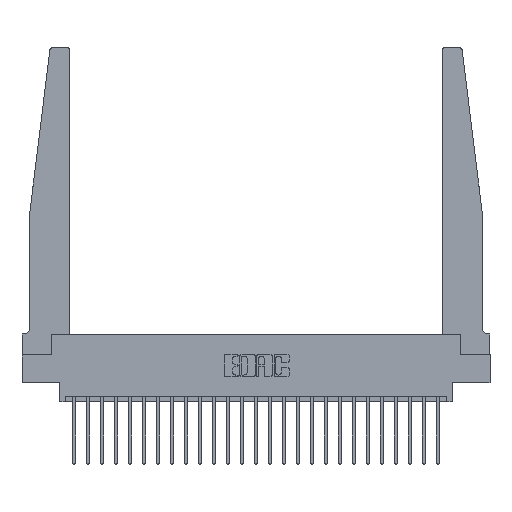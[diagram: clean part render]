
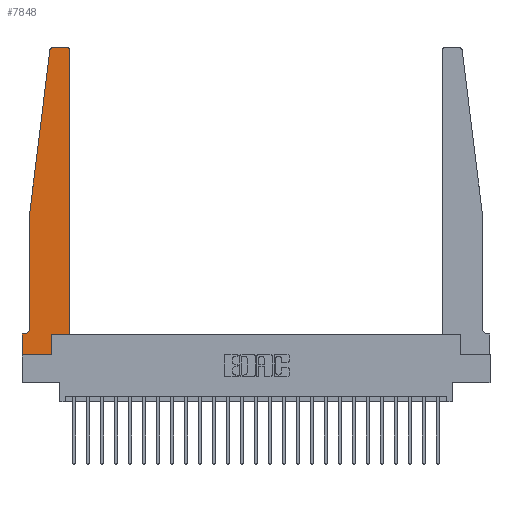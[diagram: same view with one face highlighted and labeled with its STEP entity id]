
A CAD part, top view. The second image highlights one B-rep face of the part: STEP entity #7848.
In plain terms, the highlighted planar face has unit normal (0, 0, 1).
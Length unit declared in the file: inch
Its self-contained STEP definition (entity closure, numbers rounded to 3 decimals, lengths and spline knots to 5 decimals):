
#26 = DIRECTION ( 'NONE',  ( -1., 0., 0. ) ) ;
#931 = LINE ( 'NONE', #16003, #6607 ) ;
#1035 = CARTESIAN_POINT ( 'NONE',  ( 0.065, 1.25, 0.37 ) ) ;
#1192 = VERTEX_POINT ( 'NONE', #6724 ) ;
#1644 = VERTEX_POINT ( 'NONE', #19630 ) ;
#2018 = AXIS2_PLACEMENT_3D ( 'NONE', #3687, #19014, #7598 ) ;
#2164 = CARTESIAN_POINT ( 'NONE',  ( 0.065, 0.1875, 0.37 ) ) ;
#2196 = CARTESIAN_POINT ( 'NONE',  ( 0., 0.1875, 0.37 ) ) ;
#2703 = CARTESIAN_POINT ( 'NONE',  ( 0.2605, 0.18, 0.37 ) ) ;
#3078 = VECTOR ( 'NONE', #17580, 39.37008 ) ;
#3254 = DIRECTION ( 'NONE',  ( 1., 0., 0. ) ) ;
#3283 = LINE ( 'NONE', #2164, #17925 ) ;
#3306 = CARTESIAN_POINT ( 'NONE',  ( 0.27653, 2.72, 0.37 ) ) ;
#3687 = CARTESIAN_POINT ( 'NONE',  ( 0., 0.1875, 0.37 ) ) ;
#3842 = VECTOR ( 'NONE', #23793, 39.37008 ) ;
#3896 = VERTEX_POINT ( 'NONE', #21980 ) ;
#3929 = VECTOR ( 'NONE', #10634, 39.37008 ) ;
#4028 = VERTEX_POINT ( 'NONE', #14715 ) ;
#4054 = DIRECTION ( 'NONE',  ( 0., 0., 1. ) ) ;
#4453 = ORIENTED_EDGE ( 'NONE', *, *, #22277, .T. ) ;
#4583 = CIRCLE ( 'NONE', #8729, 0.05 ) ;
#4619 = EDGE_CURVE ( 'NONE', #16346, #22479, #21189, .T. ) ;
#4813 = VERTEX_POINT ( 'NONE', #20876 ) ;
#4821 = LINE ( 'NONE', #10962, #23227 ) ;
#4935 = CIRCLE ( 'NONE', #9643, 0.03 ) ;
#4968 = CIRCLE ( 'NONE', #6593, 0.03 ) ;
#5007 = VERTEX_POINT ( 'NONE', #8241 ) ;
#5050 = ORIENTED_EDGE ( 'NONE', *, *, #11134, .T. ) ;
#5052 = ORIENTED_EDGE ( 'NONE', *, *, #17417, .T. ) ;
#5088 = CARTESIAN_POINT ( 'NONE',  ( 0.425, 2.72, 0.37 ) ) ;
#5091 = EDGE_CURVE ( 'NONE', #22479, #13939, #931, .T. ) ;
#5223 = DIRECTION ( 'NONE',  ( 1., 0., 0. ) ) ;
#5710 = CARTESIAN_POINT ( 'NONE',  ( 0.425, 0.18, 0.37 ) ) ;
#5969 = ORIENTED_EDGE ( 'NONE', *, *, #22006, .T. ) ;
#6244 = ORIENTED_EDGE ( 'NONE', *, *, #21974, .T. ) ;
#6593 = AXIS2_PLACEMENT_3D ( 'NONE', #3306, #16664, #5223 ) ;
#6607 = VECTOR ( 'NONE', #17930, 39.37008 ) ;
#6724 = CARTESIAN_POINT ( 'NONE',  ( 0.24675, 2.72367, 0.37 ) ) ;
#6766 = CARTESIAN_POINT ( 'NONE',  ( 0.2605, 0., 0.37 ) ) ;
#7598 = DIRECTION ( 'NONE',  ( 1., 0., 0. ) ) ;
#7609 = EDGE_LOOP ( 'NONE', ( #5969, #4453, #10135, #6244, #14016, #5050, #11585, #13704, #5052, #9575, #22919, #14624 ) ) ;
#7662 = VERTEX_POINT ( 'NONE', #6766 ) ;
#7848 = ADVANCED_FACE ( 'NONE', ( #11524 ), #15213, .T. ) ;
#8241 = CARTESIAN_POINT ( 'NONE',  ( 0.395, 2.75, 0.37 ) ) ;
#8729 = AXIS2_PLACEMENT_3D ( 'NONE', #22813, #11435, #26 ) ;
#9575 = ORIENTED_EDGE ( 'NONE', *, *, #4619, .T. ) ;
#9643 = AXIS2_PLACEMENT_3D ( 'NONE', #15490, #4054, #17404 ) ;
#10135 = ORIENTED_EDGE ( 'NONE', *, *, #12036, .T. ) ;
#10165 = CARTESIAN_POINT ( 'NONE',  ( 0.065, 1.25, 0.37 ) ) ;
#10360 = LINE ( 'NONE', #13999, #19884 ) ;
#10634 = DIRECTION ( 'NONE',  ( 0., 1., 0. ) ) ;
#10962 = CARTESIAN_POINT ( 'NONE',  ( 0., 0., 0.37 ) ) ;
#11134 = EDGE_CURVE ( 'NONE', #3896, #16182, #3283, .T. ) ;
#11435 = DIRECTION ( 'NONE',  ( 0., 0., -1. ) ) ;
#11524 = FACE_OUTER_BOUND ( 'NONE', #7609, .T. ) ;
#11585 = ORIENTED_EDGE ( 'NONE', *, *, #19253, .T. ) ;
#12036 = EDGE_CURVE ( 'NONE', #1192, #16999, #24025, .T. ) ;
#13704 = ORIENTED_EDGE ( 'NONE', *, *, #17629, .T. ) ;
#13939 = VERTEX_POINT ( 'NONE', #5088 ) ;
#13999 = CARTESIAN_POINT ( 'NONE',  ( 0.25, 2.75, 0.37 ) ) ;
#14016 = ORIENTED_EDGE ( 'NONE', *, *, #18045, .T. ) ;
#14624 = ORIENTED_EDGE ( 'NONE', *, *, #14674, .T. ) ;
#14674 = EDGE_CURVE ( 'NONE', #13939, #5007, #4935, .T. ) ;
#14715 = CARTESIAN_POINT ( 'NONE',  ( 0.065, 0.2375, 0.37 ) ) ;
#15213 = PLANE ( 'NONE',  #2018 ) ;
#15452 = VECTOR ( 'NONE', #15837, 39.37008 ) ;
#15490 = CARTESIAN_POINT ( 'NONE',  ( 0.395, 2.72, 0.37 ) ) ;
#15837 = DIRECTION ( 'NONE',  ( 0., -1., 0. ) ) ;
#16003 = CARTESIAN_POINT ( 'NONE',  ( 0.425, 0.18, 0.37 ) ) ;
#16024 = CARTESIAN_POINT ( 'NONE',  ( 0.065, 1.25, 0.37 ) ) ;
#16182 = VERTEX_POINT ( 'NONE', #2196 ) ;
#16346 = VERTEX_POINT ( 'NONE', #2703 ) ;
#16613 = CARTESIAN_POINT ( 'NONE',  ( 0.425, 0.18, 0.37 ) ) ;
#16664 = DIRECTION ( 'NONE',  ( 0., 0., 1. ) ) ;
#16999 = VERTEX_POINT ( 'NONE', #16024 ) ;
#17404 = DIRECTION ( 'NONE',  ( 1., 0., 0. ) ) ;
#17417 = EDGE_CURVE ( 'NONE', #7662, #16346, #19119, .T. ) ;
#17444 = DIRECTION ( 'NONE',  ( -1., 0., 0. ) ) ;
#17580 = DIRECTION ( 'NONE',  ( 1., 0., 0. ) ) ;
#17629 = EDGE_CURVE ( 'NONE', #4813, #7662, #22703, .T. ) ;
#17835 = DIRECTION ( 'NONE',  ( -1., 0., 0. ) ) ;
#17925 = VECTOR ( 'NONE', #17444, 39.37008 ) ;
#17930 = DIRECTION ( 'NONE',  ( 0., 1., 0. ) ) ;
#18045 = EDGE_CURVE ( 'NONE', #4028, #3896, #4583, .T. ) ;
#19014 = DIRECTION ( 'NONE',  ( 0., 0., 1. ) ) ;
#19119 = LINE ( 'NONE', #22762, #3929 ) ;
#19253 = EDGE_CURVE ( 'NONE', #16182, #4813, #4821, .T. ) ;
#19555 = CARTESIAN_POINT ( 'NONE',  ( 0., 0., 0.37 ) ) ;
#19630 = CARTESIAN_POINT ( 'NONE',  ( 0.27653, 2.75, 0.37 ) ) ;
#19884 = VECTOR ( 'NONE', #17835, 39.37008 ) ;
#20526 = DIRECTION ( 'NONE',  ( 0., -1., 0. ) ) ;
#20610 = VECTOR ( 'NONE', #3254, 39.37008 ) ;
#20876 = CARTESIAN_POINT ( 'NONE',  ( 0., 0., 0.37 ) ) ;
#21043 = LINE ( 'NONE', #10165, #15452 ) ;
#21189 = LINE ( 'NONE', #16613, #20610 ) ;
#21974 = EDGE_CURVE ( 'NONE', #16999, #4028, #21043, .T. ) ;
#21980 = CARTESIAN_POINT ( 'NONE',  ( 0.015, 0.1875, 0.37 ) ) ;
#22006 = EDGE_CURVE ( 'NONE', #5007, #1644, #10360, .T. ) ;
#22277 = EDGE_CURVE ( 'NONE', #1644, #1192, #4968, .T. ) ;
#22479 = VERTEX_POINT ( 'NONE', #5710 ) ;
#22703 = LINE ( 'NONE', #19555, #3078 ) ;
#22762 = CARTESIAN_POINT ( 'NONE',  ( 0.2605, 0.18, 0.37 ) ) ;
#22813 = CARTESIAN_POINT ( 'NONE',  ( 0.015, 0.2375, 0.37 ) ) ;
#22919 = ORIENTED_EDGE ( 'NONE', *, *, #5091, .T. ) ;
#23227 = VECTOR ( 'NONE', #20526, 39.37008 ) ;
#23793 = DIRECTION ( 'NONE',  ( -0.122, -0.992, 0. ) ) ;
#24025 = LINE ( 'NONE', #1035, #3842 ) ;
